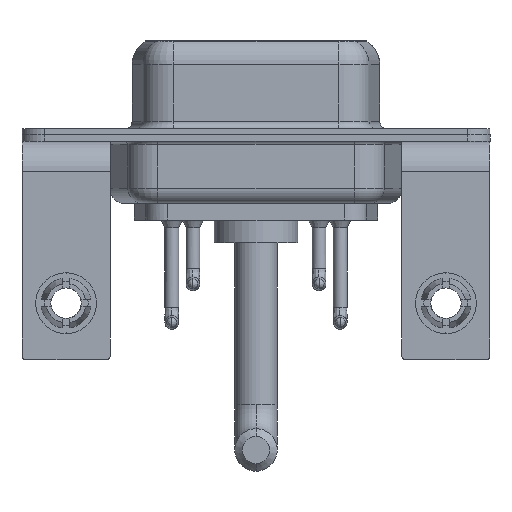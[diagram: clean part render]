
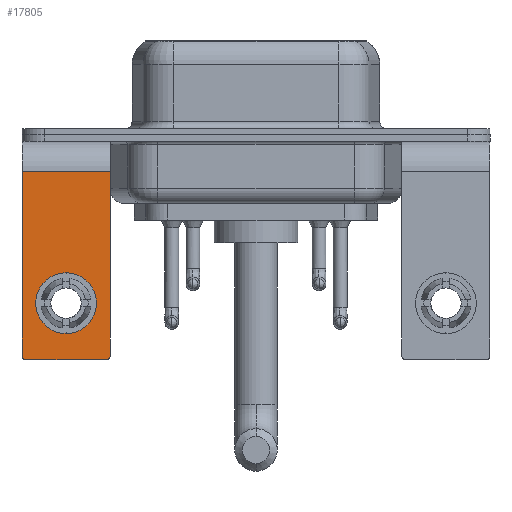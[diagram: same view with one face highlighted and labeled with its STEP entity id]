
A CAD part, front view. The second image highlights one B-rep face of the part: STEP entity #17805.
In plain terms, the highlighted planar face has unit normal (0, -1, 0).
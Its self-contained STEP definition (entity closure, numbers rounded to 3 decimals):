
#67 = CARTESIAN_POINT ( 'NONE',  ( 2.9, -6.25, -2.4 ) ) ;
#768 = CARTESIAN_POINT ( 'NONE',  ( 2.9, -6.25, -14.55 ) ) ;
#864 = FACE_OUTER_BOUND ( 'NONE', #18020, .T. ) ;
#1139 = CIRCLE ( 'NONE', #13822, 2. ) ;
#1421 = CIRCLE ( 'NONE', #6255, 0.25 ) ;
#1909 = EDGE_CURVE ( 'NONE', #10410, #14793, #10664, .T. ) ;
#1936 = CARTESIAN_POINT ( 'NONE',  ( 2.65, -6.25, -14.8 ) ) ;
#2046 = CARTESIAN_POINT ( 'NONE',  ( 2.65, -6.25, -14.55 ) ) ;
#3149 = CARTESIAN_POINT ( 'NONE',  ( -2.65, -6.25, -14.55 ) ) ;
#3727 = AXIS2_PLACEMENT_3D ( 'NONE', #9221, #6476, #9766 ) ;
#3999 = EDGE_CURVE ( 'NONE', #14525, #16600, #15179, .T. ) ;
#5042 = CARTESIAN_POINT ( 'NONE',  ( -2.9, -6.25, -14.55 ) ) ;
#5051 = CIRCLE ( 'NONE', #17101, 0.25 ) ;
#5088 = DIRECTION ( 'NONE',  ( 0., 0., 1. ) ) ;
#5187 = VERTEX_POINT ( 'NONE', #67 ) ;
#5238 = DIRECTION ( 'NONE',  ( 0., 1., 0. ) ) ;
#5299 = ORIENTED_EDGE ( 'NONE', *, *, #1909, .T. ) ;
#5390 = AXIS2_PLACEMENT_3D ( 'NONE', #18158, #5238, #10979 ) ;
#5792 = ORIENTED_EDGE ( 'NONE', *, *, #17018, .F. ) ;
#5835 = CARTESIAN_POINT ( 'NONE',  ( 0., -6.25, -11.07 ) ) ;
#6255 = AXIS2_PLACEMENT_3D ( 'NONE', #2046, #12145, #5088 ) ;
#6467 = VECTOR ( 'NONE', #12749, 1000. ) ;
#6476 = DIRECTION ( 'NONE',  ( 0., 1., 0. ) ) ;
#6654 = EDGE_CURVE ( 'NONE', #5187, #10410, #10925, .T. ) ;
#6810 = LINE ( 'NONE', #9928, #6467 ) ;
#6822 = ORIENTED_EDGE ( 'NONE', *, *, #15904, .T. ) ;
#7226 = CARTESIAN_POINT ( 'NONE',  ( 0., -6.25, -13.07 ) ) ;
#7344 = DIRECTION ( 'NONE',  ( 0., 1., 0. ) ) ;
#7939 = VERTEX_POINT ( 'NONE', #1936 ) ;
#8015 = DIRECTION ( 'NONE',  ( 0., 0., -1. ) ) ;
#8056 = FACE_BOUND ( 'NONE', #9534, .T. ) ;
#8089 = CARTESIAN_POINT ( 'NONE',  ( 2.9, -6.25, -2.4 ) ) ;
#8191 = CARTESIAN_POINT ( 'NONE',  ( 2.9, -6.25, -14.8 ) ) ;
#9101 = DIRECTION ( 'NONE',  ( 0., -1., 0. ) ) ;
#9221 = CARTESIAN_POINT ( 'NONE',  ( 0., -6.25, -11.07 ) ) ;
#9334 = DIRECTION ( 'NONE',  ( -1., 0., 0. ) ) ;
#9534 = EDGE_LOOP ( 'NONE', ( #15584, #6822 ) ) ;
#9652 = CARTESIAN_POINT ( 'NONE',  ( -2.9, -6.25, -2.4 ) ) ;
#9766 = DIRECTION ( 'NONE',  ( 0., 0., 1. ) ) ;
#9862 = CARTESIAN_POINT ( 'NONE',  ( -2.65, -6.25, -14.8 ) ) ;
#9928 = CARTESIAN_POINT ( 'NONE',  ( 2.9, -6.25, -2.4 ) ) ;
#10044 = ORIENTED_EDGE ( 'NONE', *, *, #14241, .T. ) ;
#10305 = ORIENTED_EDGE ( 'NONE', *, *, #13245, .T. ) ;
#10410 = VERTEX_POINT ( 'NONE', #9652 ) ;
#10423 = EDGE_CURVE ( 'NONE', #5187, #17733, #6810, .T. ) ;
#10483 = CARTESIAN_POINT ( 'NONE',  ( -2.9, -6.25, -2.4 ) ) ;
#10664 = LINE ( 'NONE', #10483, #16242 ) ;
#10925 = LINE ( 'NONE', #8089, #10936 ) ;
#10936 = VECTOR ( 'NONE', #11193, 1000. ) ;
#10957 = CARTESIAN_POINT ( 'NONE',  ( 0., -6.25, -9.07 ) ) ;
#10979 = DIRECTION ( 'NONE',  ( 0., 0., 1. ) ) ;
#11193 = DIRECTION ( 'NONE',  ( -1., 0., 0. ) ) ;
#12145 = DIRECTION ( 'NONE',  ( 0., -1., 0. ) ) ;
#12390 = PLANE ( 'NONE',  #5390 ) ;
#12749 = DIRECTION ( 'NONE',  ( 0., 0., -1. ) ) ;
#12997 = DIRECTION ( 'NONE',  ( 0., 0., 1. ) ) ;
#13059 = DIRECTION ( 'NONE',  ( 0., 0., 1. ) ) ;
#13245 = EDGE_CURVE ( 'NONE', #14793, #14515, #5051, .T. ) ;
#13822 = AXIS2_PLACEMENT_3D ( 'NONE', #5835, #7344, #12997 ) ;
#14161 = ORIENTED_EDGE ( 'NONE', *, *, #10423, .F. ) ;
#14241 = EDGE_CURVE ( 'NONE', #7939, #17733, #1421, .T. ) ;
#14515 = VERTEX_POINT ( 'NONE', #9862 ) ;
#14525 = VERTEX_POINT ( 'NONE', #7226 ) ;
#14793 = VERTEX_POINT ( 'NONE', #5042 ) ;
#15179 = CIRCLE ( 'NONE', #3727, 2. ) ;
#15293 = VECTOR ( 'NONE', #9334, 1000. ) ;
#15584 = ORIENTED_EDGE ( 'NONE', *, *, #3999, .T. ) ;
#15904 = EDGE_CURVE ( 'NONE', #16600, #14525, #1139, .T. ) ;
#16242 = VECTOR ( 'NONE', #8015, 1000. ) ;
#16482 = LINE ( 'NONE', #8191, #15293 ) ;
#16600 = VERTEX_POINT ( 'NONE', #10957 ) ;
#17018 = EDGE_CURVE ( 'NONE', #7939, #14515, #16482, .T. ) ;
#17101 = AXIS2_PLACEMENT_3D ( 'NONE', #3149, #9101, #13059 ) ;
#17191 = ORIENTED_EDGE ( 'NONE', *, *, #6654, .T. ) ;
#17733 = VERTEX_POINT ( 'NONE', #768 ) ;
#17805 = ADVANCED_FACE ( 'NONE', ( #8056, #864 ), #12390, .F. ) ;
#18020 = EDGE_LOOP ( 'NONE', ( #5299, #10305, #5792, #10044, #14161, #17191 ) ) ;
#18158 = CARTESIAN_POINT ( 'NONE',  ( 2.9, -6.25, -2.4 ) ) ;
